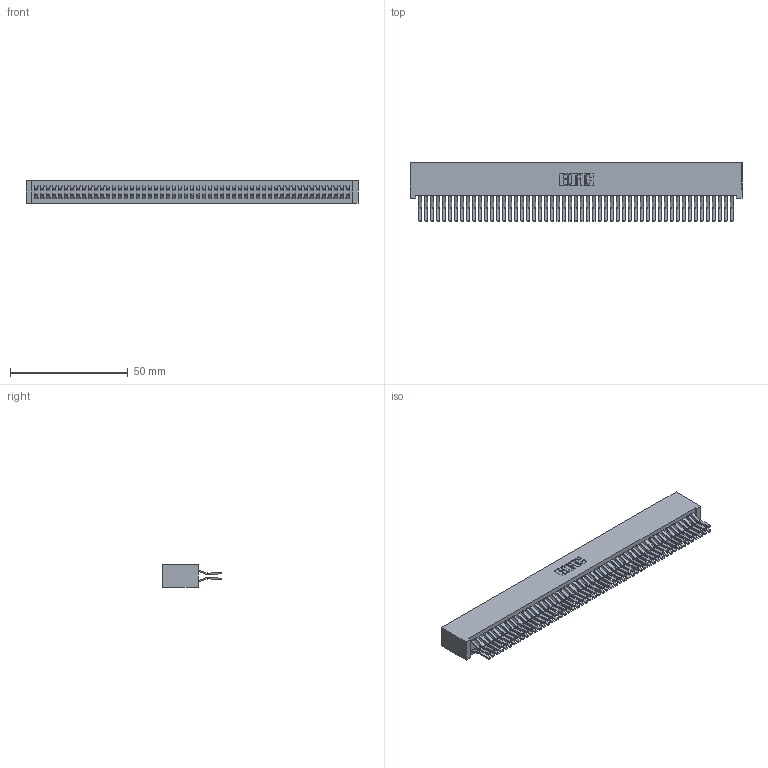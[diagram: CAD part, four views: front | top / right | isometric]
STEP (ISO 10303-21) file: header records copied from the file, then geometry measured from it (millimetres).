
FILE_DESCRIPTION (( 'STEP AP203' ), '1' );
FILE_NAME ('392-106-560-201.STEP', '2018-08-18T20:39:44', ( '' ), ( '' ), 'SwSTEP 2.0', 'SolidWorks 2016', '' );
FILE_SCHEMA (( 'CONFIG_CONTROL_DESIGN' ));
Length unit declared in the file: inch
Products named in the file (3): 342 Part_Lugless; 345-292-001_560 Tail; 392-106-560-201
Assembly tree (107 placements, depth 2):
  392-106-560-201
    342 Part_Lugless
    345-292-001_560 Tail  x106
Bounding box: 140.87 x 24.78 x 9.4 mm (x, y, z)
Volume: 13844.5 mm3; surface area: 24921.4 mm2
Topology: 107 solids, 107 shells, 5826 faces, 17341 edges, 11418 vertices
Faces by surface type: plane 3878, cylinder 1948
Entity records: 32353 total; most frequent: CARTESIAN_POINT 5346, ORIENTED_EDGE 5282, DIRECTION 4545, EDGE_CURVE 2641, VECTOR 2517, LINE 2517, VERTEX_POINT 1758, AXIS2_PLACEMENT_3D 1014
